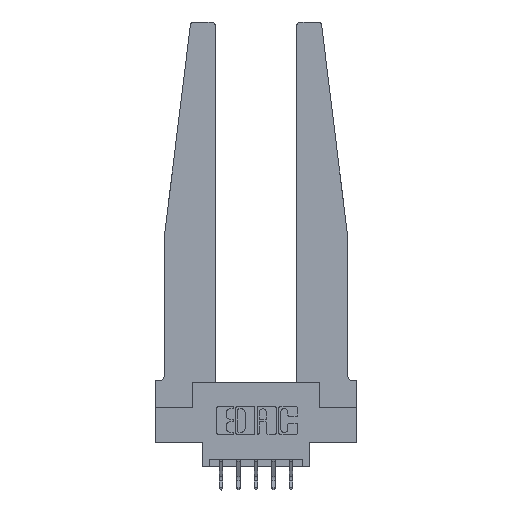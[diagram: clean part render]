
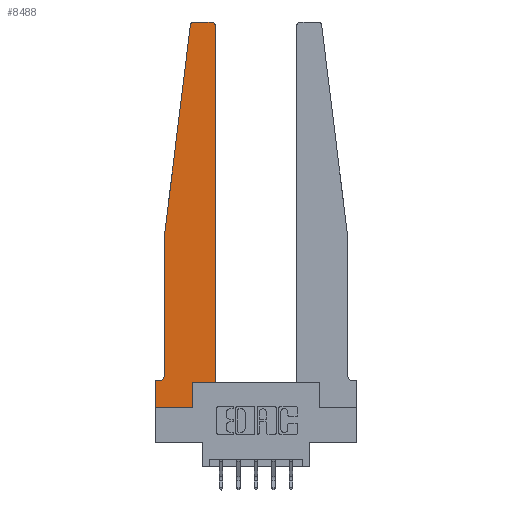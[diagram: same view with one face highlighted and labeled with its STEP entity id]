
A CAD part, top view. The second image highlights one B-rep face of the part: STEP entity #8488.
In plain terms, the highlighted planar face has unit normal (0, 0, 1).
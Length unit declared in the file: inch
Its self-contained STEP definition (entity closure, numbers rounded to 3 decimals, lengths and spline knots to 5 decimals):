
#200 = DIRECTION ( 'NONE',  ( 1., 0., 0. ) ) ;
#245 = LINE ( 'NONE', #12567, #2359 ) ;
#426 = CARTESIAN_POINT ( 'NONE',  ( 0.425, 2.72, 0.37 ) ) ;
#455 = EDGE_CURVE ( 'NONE', #10319, #3315, #12366, .T. ) ;
#613 = EDGE_CURVE ( 'NONE', #12720, #615, #2190, .T. ) ;
#615 = VERTEX_POINT ( 'NONE', #4104 ) ;
#798 = EDGE_CURVE ( 'NONE', #7444, #8866, #245, .T. ) ;
#832 = VECTOR ( 'NONE', #8476, 39.37008 ) ;
#1239 = LINE ( 'NONE', #9241, #6403 ) ;
#1691 = ORIENTED_EDGE ( 'NONE', *, *, #8056, .T. ) ;
#2059 = LINE ( 'NONE', #2467, #4491 ) ;
#2190 = LINE ( 'NONE', #6122, #12841 ) ;
#2298 = CARTESIAN_POINT ( 'NONE',  ( 0.015, 0.1875, 0.37 ) ) ;
#2359 = VECTOR ( 'NONE', #200, 39.37008 ) ;
#2414 = ORIENTED_EDGE ( 'NONE', *, *, #9885, .T. ) ;
#2467 = CARTESIAN_POINT ( 'NONE',  ( 0.065, 1.25, 0.37 ) ) ;
#2508 = DIRECTION ( 'NONE',  ( -0.122, -0.992, 0. ) ) ;
#2516 = VERTEX_POINT ( 'NONE', #13258 ) ;
#2641 = VECTOR ( 'NONE', #8617, 39.37008 ) ;
#2835 = DIRECTION ( 'NONE',  ( 0., -1., 0. ) ) ;
#3001 = PLANE ( 'NONE',  #8092 ) ;
#3315 = VERTEX_POINT ( 'NONE', #7300 ) ;
#3503 = CARTESIAN_POINT ( 'NONE',  ( 0.24675, 2.72367, 0.37 ) ) ;
#3916 = CIRCLE ( 'NONE', #4899, 0.03 ) ;
#4045 = DIRECTION ( 'NONE',  ( 1., 0., 0. ) ) ;
#4079 = VERTEX_POINT ( 'NONE', #426 ) ;
#4104 = CARTESIAN_POINT ( 'NONE',  ( 0., 0.1875, 0.37 ) ) ;
#4373 = CARTESIAN_POINT ( 'NONE',  ( 0.425, 0.18, 0.37 ) ) ;
#4384 = AXIS2_PLACEMENT_3D ( 'NONE', #11598, #5438, #12639 ) ;
#4476 = CARTESIAN_POINT ( 'NONE',  ( 0.395, 2.72, 0.37 ) ) ;
#4491 = VECTOR ( 'NONE', #2508, 39.37008 ) ;
#4559 = CARTESIAN_POINT ( 'NONE',  ( 0., 0., 0.37 ) ) ;
#4595 = DIRECTION ( 'NONE',  ( 0., 1., 0. ) ) ;
#4717 = CIRCLE ( 'NONE', #4384, 0.05 ) ;
#4899 = AXIS2_PLACEMENT_3D ( 'NONE', #11568, #5409, #12609 ) ;
#5371 = EDGE_CURVE ( 'NONE', #615, #7444, #13211, .T. ) ;
#5409 = DIRECTION ( 'NONE',  ( 0., 0., 1. ) ) ;
#5438 = DIRECTION ( 'NONE',  ( 0., 0., -1. ) ) ;
#5508 = DIRECTION ( 'NONE',  ( 1., 0., 0. ) ) ;
#5579 = CARTESIAN_POINT ( 'NONE',  ( 0.2605, 0.18, 0.37 ) ) ;
#5641 = ORIENTED_EDGE ( 'NONE', *, *, #8685, .T. ) ;
#5725 = ORIENTED_EDGE ( 'NONE', *, *, #7165, .T. ) ;
#6021 = CARTESIAN_POINT ( 'NONE',  ( 0., 0., 0.37 ) ) ;
#6122 = CARTESIAN_POINT ( 'NONE',  ( 0.065, 0.1875, 0.37 ) ) ;
#6377 = ORIENTED_EDGE ( 'NONE', *, *, #11678, .T. ) ;
#6403 = VECTOR ( 'NONE', #10262, 39.37008 ) ;
#6428 = CARTESIAN_POINT ( 'NONE',  ( 0.27653, 2.75, 0.37 ) ) ;
#6625 = AXIS2_PLACEMENT_3D ( 'NONE', #4476, #11666, #5508 ) ;
#7165 = EDGE_CURVE ( 'NONE', #9928, #11850, #8132, .T. ) ;
#7232 = CARTESIAN_POINT ( 'NONE',  ( 0.065, 1.25, 0.37 ) ) ;
#7300 = CARTESIAN_POINT ( 'NONE',  ( 0.065, 0.2375, 0.37 ) ) ;
#7444 = VERTEX_POINT ( 'NONE', #6021 ) ;
#7603 = FACE_OUTER_BOUND ( 'NONE', #11166, .T. ) ;
#7856 = CARTESIAN_POINT ( 'NONE',  ( 0.2605, 0., 0.37 ) ) ;
#7934 = CARTESIAN_POINT ( 'NONE',  ( 0.065, 1.25, 0.37 ) ) ;
#8056 = EDGE_CURVE ( 'NONE', #11584, #8156, #3916, .T. ) ;
#8061 = EDGE_CURVE ( 'NONE', #11850, #4079, #11813, .T. ) ;
#8092 = AXIS2_PLACEMENT_3D ( 'NONE', #12240, #10225, #4045 ) ;
#8132 = LINE ( 'NONE', #8529, #2641 ) ;
#8156 = VERTEX_POINT ( 'NONE', #3503 ) ;
#8476 = DIRECTION ( 'NONE',  ( 0., 1., 0. ) ) ;
#8488 = ADVANCED_FACE ( 'NONE', ( #7603 ), #3001, .T. ) ;
#8529 = CARTESIAN_POINT ( 'NONE',  ( 0.425, 0.18, 0.37 ) ) ;
#8617 = DIRECTION ( 'NONE',  ( 1., 0., 0. ) ) ;
#8685 = EDGE_CURVE ( 'NONE', #3315, #12720, #4717, .T. ) ;
#8748 = CARTESIAN_POINT ( 'NONE',  ( 0.2605, 0.18, 0.37 ) ) ;
#8866 = VERTEX_POINT ( 'NONE', #7856 ) ;
#9241 = CARTESIAN_POINT ( 'NONE',  ( 0.25, 2.75, 0.37 ) ) ;
#9307 = EDGE_CURVE ( 'NONE', #4079, #2516, #9543, .T. ) ;
#9329 = VECTOR ( 'NONE', #2835, 39.37008 ) ;
#9422 = ORIENTED_EDGE ( 'NONE', *, *, #8061, .T. ) ;
#9543 = CIRCLE ( 'NONE', #6625, 0.03 ) ;
#9885 = EDGE_CURVE ( 'NONE', #8866, #9928, #13373, .T. ) ;
#9928 = VERTEX_POINT ( 'NONE', #8748 ) ;
#10161 = VECTOR ( 'NONE', #11755, 39.37008 ) ;
#10225 = DIRECTION ( 'NONE',  ( 0., 0., 1. ) ) ;
#10262 = DIRECTION ( 'NONE',  ( -1., 0., 0. ) ) ;
#10283 = DIRECTION ( 'NONE',  ( -1., 0., 0. ) ) ;
#10319 = VERTEX_POINT ( 'NONE', #7232 ) ;
#10627 = VECTOR ( 'NONE', #4595, 39.37008 ) ;
#10650 = ORIENTED_EDGE ( 'NONE', *, *, #798, .T. ) ;
#10978 = CARTESIAN_POINT ( 'NONE',  ( 0.425, 0.18, 0.37 ) ) ;
#11155 = ORIENTED_EDGE ( 'NONE', *, *, #12041, .T. ) ;
#11166 = EDGE_LOOP ( 'NONE', ( #11155, #1691, #6377, #12777, #5641, #12052, #11197, #10650, #2414, #5725, #9422, #12209 ) ) ;
#11197 = ORIENTED_EDGE ( 'NONE', *, *, #5371, .T. ) ;
#11568 = CARTESIAN_POINT ( 'NONE',  ( 0.27653, 2.72, 0.37 ) ) ;
#11584 = VERTEX_POINT ( 'NONE', #6428 ) ;
#11598 = CARTESIAN_POINT ( 'NONE',  ( 0.015, 0.2375, 0.37 ) ) ;
#11666 = DIRECTION ( 'NONE',  ( 0., 0., 1. ) ) ;
#11678 = EDGE_CURVE ( 'NONE', #8156, #10319, #2059, .T. ) ;
#11755 = DIRECTION ( 'NONE',  ( 0., -1., 0. ) ) ;
#11813 = LINE ( 'NONE', #4373, #832 ) ;
#11850 = VERTEX_POINT ( 'NONE', #10978 ) ;
#12041 = EDGE_CURVE ( 'NONE', #2516, #11584, #1239, .T. ) ;
#12052 = ORIENTED_EDGE ( 'NONE', *, *, #613, .T. ) ;
#12209 = ORIENTED_EDGE ( 'NONE', *, *, #9307, .T. ) ;
#12240 = CARTESIAN_POINT ( 'NONE',  ( 0., 0.1875, 0.37 ) ) ;
#12366 = LINE ( 'NONE', #7934, #9329 ) ;
#12567 = CARTESIAN_POINT ( 'NONE',  ( 0., 0., 0.37 ) ) ;
#12609 = DIRECTION ( 'NONE',  ( 1., 0., 0. ) ) ;
#12639 = DIRECTION ( 'NONE',  ( -1., 0., 0. ) ) ;
#12720 = VERTEX_POINT ( 'NONE', #2298 ) ;
#12777 = ORIENTED_EDGE ( 'NONE', *, *, #455, .T. ) ;
#12841 = VECTOR ( 'NONE', #10283, 39.37008 ) ;
#13211 = LINE ( 'NONE', #4559, #10161 ) ;
#13258 = CARTESIAN_POINT ( 'NONE',  ( 0.395, 2.75, 0.37 ) ) ;
#13373 = LINE ( 'NONE', #5579, #10627 ) ;
